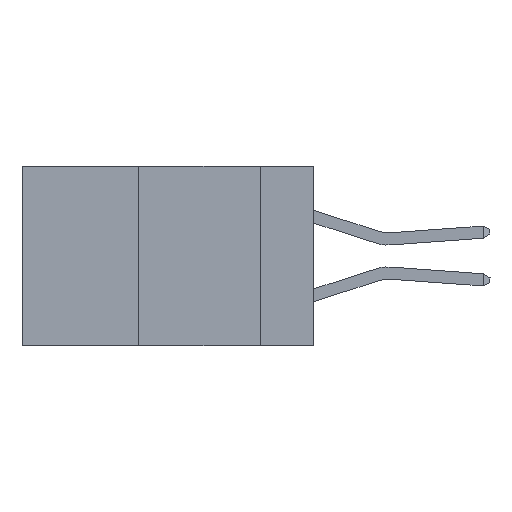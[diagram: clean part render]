
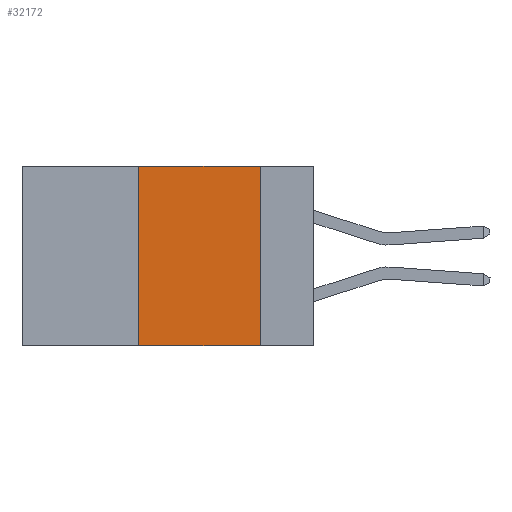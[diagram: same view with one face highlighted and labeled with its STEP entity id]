
A CAD part, left-side view. The second image highlights one B-rep face of the part: STEP entity #32172.
In plain terms, the highlighted planar face has unit normal (-1, 0, 0).
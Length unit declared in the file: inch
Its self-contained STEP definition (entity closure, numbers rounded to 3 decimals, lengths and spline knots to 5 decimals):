
#170 = ORIENTED_EDGE ( 'NONE', *, *, #6839, .F. ) ;
#177 = VERTEX_POINT ( 'NONE', #8769 ) ;
#609 = VECTOR ( 'NONE', #23155, 39.37008 ) ;
#1185 = VECTOR ( 'NONE', #32216, 39.37008 ) ;
#2725 = CARTESIAN_POINT ( 'NONE',  ( 0., 0.6, 0. ) ) ;
#2945 = DIRECTION ( 'NONE',  ( 0., -1., 0. ) ) ;
#3507 = DIRECTION ( 'NONE',  ( 0., 0., -1. ) ) ;
#4423 = VERTEX_POINT ( 'NONE', #8759 ) ;
#4818 = EDGE_CURVE ( 'NONE', #4423, #8307, #12141, .T. ) ;
#5223 = LINE ( 'NONE', #6910, #609 ) ;
#5307 = EDGE_CURVE ( 'NONE', #177, #27941, #30799, .T. ) ;
#5644 = PLANE ( 'NONE',  #11045 ) ;
#6839 = EDGE_CURVE ( 'NONE', #27941, #8307, #5223, .T. ) ;
#6910 = CARTESIAN_POINT ( 'NONE',  ( 0., 0.11, 0. ) ) ;
#8307 = VERTEX_POINT ( 'NONE', #30581 ) ;
#8759 = CARTESIAN_POINT ( 'NONE',  ( 0., 0.36, -0.37 ) ) ;
#8769 = CARTESIAN_POINT ( 'NONE',  ( 0., 0.36, 0. ) ) ;
#11045 = AXIS2_PLACEMENT_3D ( 'NONE', #30184, #27536, #3507 ) ;
#11579 = ORIENTED_EDGE ( 'NONE', *, *, #31776, .F. ) ;
#12141 = LINE ( 'NONE', #29380, #1185 ) ;
#13142 = FACE_OUTER_BOUND ( 'NONE', #32753, .T. ) ;
#14401 = LINE ( 'NONE', #28652, #26742 ) ;
#14989 = DIRECTION ( 'NONE',  ( 0., 0., 1. ) ) ;
#16700 = ORIENTED_EDGE ( 'NONE', *, *, #4818, .T. ) ;
#18055 = VECTOR ( 'NONE', #2945, 39.37008 ) ;
#23155 = DIRECTION ( 'NONE',  ( 0., 0., -1. ) ) ;
#26292 = ORIENTED_EDGE ( 'NONE', *, *, #5307, .F. ) ;
#26742 = VECTOR ( 'NONE', #14989, 39.37008 ) ;
#27536 = DIRECTION ( 'NONE',  ( 1., 0., 0. ) ) ;
#27941 = VERTEX_POINT ( 'NONE', #29780 ) ;
#28652 = CARTESIAN_POINT ( 'NONE',  ( 0., 0.36, 0. ) ) ;
#29380 = CARTESIAN_POINT ( 'NONE',  ( 0., 0.6, -0.37 ) ) ;
#29780 = CARTESIAN_POINT ( 'NONE',  ( 0., 0.11, 0. ) ) ;
#30184 = CARTESIAN_POINT ( 'NONE',  ( 0., 0.6, 0. ) ) ;
#30581 = CARTESIAN_POINT ( 'NONE',  ( 0., 0.11, -0.37 ) ) ;
#30799 = LINE ( 'NONE', #2725, #18055 ) ;
#31776 = EDGE_CURVE ( 'NONE', #4423, #177, #14401, .T. ) ;
#32172 = ADVANCED_FACE ( 'NONE', ( #13142 ), #5644, .F. ) ;
#32216 = DIRECTION ( 'NONE',  ( 0., -1., 0. ) ) ;
#32753 = EDGE_LOOP ( 'NONE', ( #170, #26292, #11579, #16700 ) ) ;
